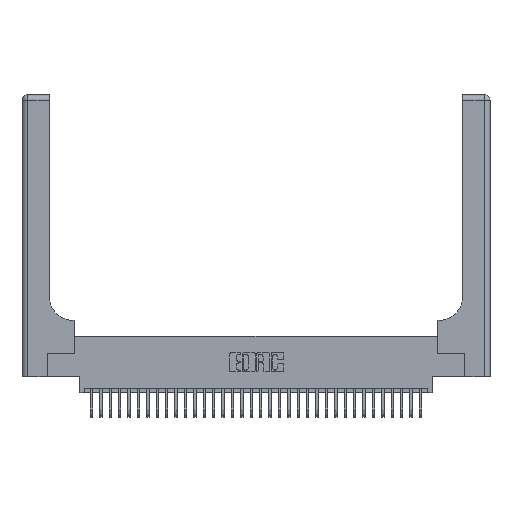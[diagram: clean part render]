
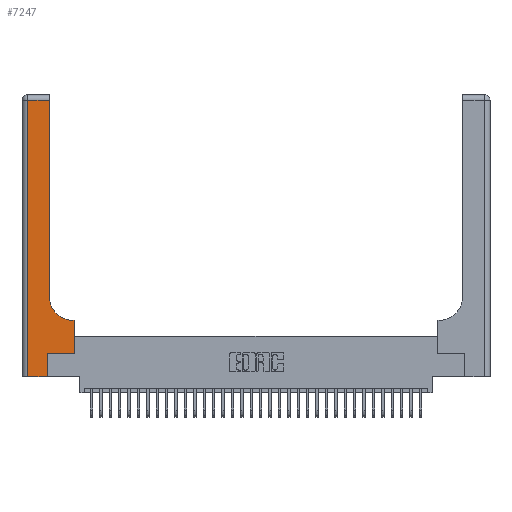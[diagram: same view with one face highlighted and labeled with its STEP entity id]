
A CAD part, top view. The second image highlights one B-rep face of the part: STEP entity #7247.
In plain terms, the highlighted planar face has unit normal (0, 0, 1).
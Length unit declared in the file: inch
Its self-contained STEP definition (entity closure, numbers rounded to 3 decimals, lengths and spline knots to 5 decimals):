
#495 = DIRECTION ( 'NONE',  ( 0., 1., 0. ) ) ;
#897 = ORIENTED_EDGE ( 'NONE', *, *, #21975, .T. ) ;
#1162 = DIRECTION ( 'NONE',  ( 0., 1., 0. ) ) ;
#1172 = VECTOR ( 'NONE', #14910, 39.37008 ) ;
#1519 = DIRECTION ( 'NONE',  ( 0., -1., 0. ) ) ;
#1652 = DIRECTION ( 'NONE',  ( 1., 0., 0. ) ) ;
#2451 = VERTEX_POINT ( 'NONE', #6832 ) ;
#2581 = VERTEX_POINT ( 'NONE', #22828 ) ;
#2942 = VECTOR ( 'NONE', #5007, 39.37008 ) ;
#3755 = CARTESIAN_POINT ( 'NONE',  ( 0.2915, 3., 0.37 ) ) ;
#3783 = CARTESIAN_POINT ( 'NONE',  ( 0.269, 0., 0.37 ) ) ;
#3877 = EDGE_CURVE ( 'NONE', #33145, #2581, #27652, .T. ) ;
#4022 = CARTESIAN_POINT ( 'NONE',  ( 0.5415, 0.6, 0.37 ) ) ;
#4668 = CARTESIAN_POINT ( 'NONE',  ( 0.2915, 0.6, 0.37 ) ) ;
#5007 = DIRECTION ( 'NONE',  ( -1., 0., 0. ) ) ;
#5015 = CARTESIAN_POINT ( 'NONE',  ( 0.269, 0., 0.37 ) ) ;
#5413 = CARTESIAN_POINT ( 'NONE',  ( 0.269, 0.25, 0.37 ) ) ;
#5537 = EDGE_CURVE ( 'NONE', #2581, #27864, #6064, .T. ) ;
#5750 = ORIENTED_EDGE ( 'NONE', *, *, #7072, .T. ) ;
#6064 = LINE ( 'NONE', #9080, #25805 ) ;
#6149 = VECTOR ( 'NONE', #1162, 39.37008 ) ;
#6354 = VECTOR ( 'NONE', #495, 39.37008 ) ;
#6381 = ORIENTED_EDGE ( 'NONE', *, *, #17671, .T. ) ;
#6402 = VERTEX_POINT ( 'NONE', #10363 ) ;
#6479 = PLANE ( 'NONE',  #25214 ) ;
#6832 = CARTESIAN_POINT ( 'NONE',  ( 0.2915, 2.94, 0.37 ) ) ;
#6835 = VERTEX_POINT ( 'NONE', #32559 ) ;
#7072 = EDGE_CURVE ( 'NONE', #6402, #6835, #26923, .T. ) ;
#7247 = ADVANCED_FACE ( 'NONE', ( #15195 ), #6479, .F. ) ;
#7998 = DIRECTION ( 'NONE',  ( 1., 0., 0. ) ) ;
#8731 = EDGE_LOOP ( 'NONE', ( #897, #13013, #22154, #17808, #6381, #12710, #5750, #23769, #18027 ) ) ;
#9080 = CARTESIAN_POINT ( 'NONE',  ( 0., 0., 0.37 ) ) ;
#10363 = CARTESIAN_POINT ( 'NONE',  ( 0.5585, 0.25, 0.37 ) ) ;
#10382 = CARTESIAN_POINT ( 'NONE',  ( 0.269, 0.25, 0.37 ) ) ;
#11496 = VECTOR ( 'NONE', #1519, 39.37008 ) ;
#11647 = DIRECTION ( 'NONE',  ( 0., 0., -1. ) ) ;
#11668 = DIRECTION ( 'NONE',  ( 1., 0., 0. ) ) ;
#12370 = LINE ( 'NONE', #5413, #18421 ) ;
#12710 = ORIENTED_EDGE ( 'NONE', *, *, #18711, .T. ) ;
#13013 = ORIENTED_EDGE ( 'NONE', *, *, #21600, .T. ) ;
#14910 = DIRECTION ( 'NONE',  ( -1., 0., 0. ) ) ;
#15195 = FACE_OUTER_BOUND ( 'NONE', #8731, .T. ) ;
#15933 = CARTESIAN_POINT ( 'NONE',  ( 0.5585, 0.25, 0.37 ) ) ;
#17106 = DIRECTION ( 'NONE',  ( 0., 0., -1. ) ) ;
#17107 = EDGE_CURVE ( 'NONE', #21318, #18096, #27414, .T. ) ;
#17671 = EDGE_CURVE ( 'NONE', #27864, #26777, #29370, .T. ) ;
#17808 = ORIENTED_EDGE ( 'NONE', *, *, #5537, .T. ) ;
#18027 = ORIENTED_EDGE ( 'NONE', *, *, #17107, .T. ) ;
#18096 = VERTEX_POINT ( 'NONE', #26068 ) ;
#18421 = VECTOR ( 'NONE', #7998, 39.37008 ) ;
#18711 = EDGE_CURVE ( 'NONE', #26777, #6402, #12370, .T. ) ;
#19880 = LINE ( 'NONE', #3755, #6149 ) ;
#21318 = VERTEX_POINT ( 'NONE', #4022 ) ;
#21600 = EDGE_CURVE ( 'NONE', #2451, #33145, #22699, .T. ) ;
#21975 = EDGE_CURVE ( 'NONE', #18096, #2451, #19880, .T. ) ;
#22154 = ORIENTED_EDGE ( 'NONE', *, *, #3877, .T. ) ;
#22532 = VECTOR ( 'NONE', #26993, 39.37008 ) ;
#22699 = LINE ( 'NONE', #28220, #2942 ) ;
#22828 = CARTESIAN_POINT ( 'NONE',  ( 0.06, 0., 0.37 ) ) ;
#23769 = ORIENTED_EDGE ( 'NONE', *, *, #24566, .T. ) ;
#24566 = EDGE_CURVE ( 'NONE', #6835, #21318, #28578, .T. ) ;
#24659 = CARTESIAN_POINT ( 'NONE',  ( 0.06, 2.94, 0.37 ) ) ;
#25214 = AXIS2_PLACEMENT_3D ( 'NONE', #32100, #11647, #29668 ) ;
#25805 = VECTOR ( 'NONE', #11668, 39.37008 ) ;
#26068 = CARTESIAN_POINT ( 'NONE',  ( 0.2915, 0.85, 0.37 ) ) ;
#26777 = VERTEX_POINT ( 'NONE', #10382 ) ;
#26923 = LINE ( 'NONE', #15933, #6354 ) ;
#26993 = DIRECTION ( 'NONE',  ( 0., 1., 0. ) ) ;
#27217 = CARTESIAN_POINT ( 'NONE',  ( 0.06, 3., 0.37 ) ) ;
#27414 = CIRCLE ( 'NONE', #31146, 0.25 ) ;
#27652 = LINE ( 'NONE', #27217, #11496 ) ;
#27864 = VERTEX_POINT ( 'NONE', #5015 ) ;
#28220 = CARTESIAN_POINT ( 'NONE',  ( 0., 2.94, 0.37 ) ) ;
#28578 = LINE ( 'NONE', #4668, #1172 ) ;
#29370 = LINE ( 'NONE', #3783, #22532 ) ;
#29668 = DIRECTION ( 'NONE',  ( -1., 0., 0. ) ) ;
#31146 = AXIS2_PLACEMENT_3D ( 'NONE', #32465, #17106, #1652 ) ;
#32100 = CARTESIAN_POINT ( 'NONE',  ( 0., 3., 0.37 ) ) ;
#32465 = CARTESIAN_POINT ( 'NONE',  ( 0.5415, 0.85, 0.37 ) ) ;
#32559 = CARTESIAN_POINT ( 'NONE',  ( 0.5585, 0.6, 0.37 ) ) ;
#33145 = VERTEX_POINT ( 'NONE', #24659 ) ;
